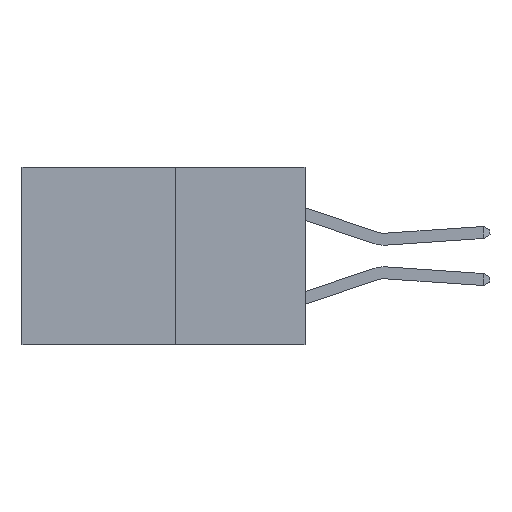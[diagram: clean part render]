
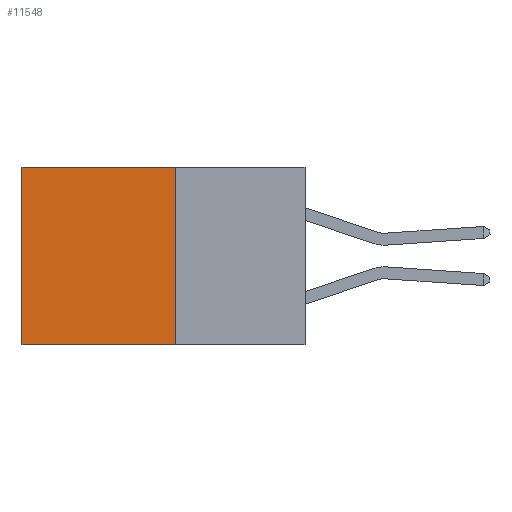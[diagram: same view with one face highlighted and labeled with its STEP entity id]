
A CAD part, left-side view. The second image highlights one B-rep face of the part: STEP entity #11548.
In plain terms, the highlighted planar face has unit normal (-1, 0, 0).
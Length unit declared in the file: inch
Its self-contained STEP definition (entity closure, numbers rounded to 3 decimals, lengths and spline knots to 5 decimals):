
#1193 = ORIENTED_EDGE ( 'NONE', *, *, #15626, .T. ) ;
#1995 = LINE ( 'NONE', #26670, #22821 ) ;
#3006 = CARTESIAN_POINT ( 'NONE',  ( 0.277, 0.27, -0.37 ) ) ;
#4322 = EDGE_CURVE ( 'NONE', #8184, #12661, #5105, .T. ) ;
#5105 = LINE ( 'NONE', #8123, #26655 ) ;
#5799 = DIRECTION ( 'NONE',  ( 0., 0., -1. ) ) ;
#8039 = AXIS2_PLACEMENT_3D ( 'NONE', #3006, #22019, #5799 ) ;
#8123 = CARTESIAN_POINT ( 'NONE',  ( 0.277, 0.59, -0.37 ) ) ;
#8184 = VERTEX_POINT ( 'NONE', #26989 ) ;
#8212 = DIRECTION ( 'NONE',  ( 0., 0., -1. ) ) ;
#10819 = VECTOR ( 'NONE', #12412, 39.37008 ) ;
#11548 = ADVANCED_FACE ( 'NONE', ( #15783 ), #21907, .F. ) ;
#12412 = DIRECTION ( 'NONE',  ( 0., 1., 0. ) ) ;
#12661 = VERTEX_POINT ( 'NONE', #23572 ) ;
#14712 = ORIENTED_EDGE ( 'NONE', *, *, #4322, .T. ) ;
#15626 = EDGE_CURVE ( 'NONE', #25633, #8184, #17146, .T. ) ;
#15783 = FACE_OUTER_BOUND ( 'NONE', #20976, .T. ) ;
#17146 = LINE ( 'NONE', #31117, #10819 ) ;
#17286 = ORIENTED_EDGE ( 'NONE', *, *, #20559, .F. ) ;
#18550 = CARTESIAN_POINT ( 'NONE',  ( 0.277, 0.27, -0.37 ) ) ;
#20559 = EDGE_CURVE ( 'NONE', #25633, #29410, #1995, .T. ) ;
#20976 = EDGE_LOOP ( 'NONE', ( #14712, #23703, #17286, #1193 ) ) ;
#21907 = PLANE ( 'NONE',  #8039 ) ;
#22019 = DIRECTION ( 'NONE',  ( 1., 0., 0. ) ) ;
#22821 = VECTOR ( 'NONE', #29358, 39.37008 ) ;
#23572 = CARTESIAN_POINT ( 'NONE',  ( 0.277, 0.59, -0.37 ) ) ;
#23703 = ORIENTED_EDGE ( 'NONE', *, *, #30148, .F. ) ;
#24968 = CARTESIAN_POINT ( 'NONE',  ( 0.277, 0.27, 0. ) ) ;
#25633 = VERTEX_POINT ( 'NONE', #24968 ) ;
#26240 = VECTOR ( 'NONE', #29192, 39.37008 ) ;
#26655 = VECTOR ( 'NONE', #8212, 39.37008 ) ;
#26670 = CARTESIAN_POINT ( 'NONE',  ( 0.277, 0.27, -0.37 ) ) ;
#26989 = CARTESIAN_POINT ( 'NONE',  ( 0.277, 0.59, 0. ) ) ;
#27090 = LINE ( 'NONE', #18550, #26240 ) ;
#29192 = DIRECTION ( 'NONE',  ( 0., 1., 0. ) ) ;
#29358 = DIRECTION ( 'NONE',  ( 0., 0., -1. ) ) ;
#29410 = VERTEX_POINT ( 'NONE', #32719 ) ;
#30148 = EDGE_CURVE ( 'NONE', #29410, #12661, #27090, .T. ) ;
#31117 = CARTESIAN_POINT ( 'NONE',  ( 0.277, 0.27, 0. ) ) ;
#32719 = CARTESIAN_POINT ( 'NONE',  ( 0.277, 0.27, -0.37 ) ) ;
